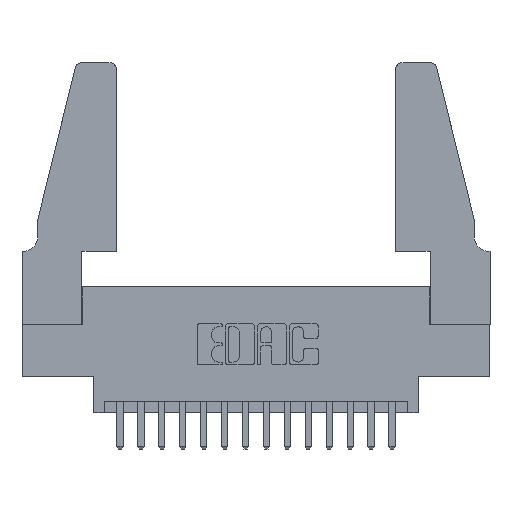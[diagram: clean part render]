
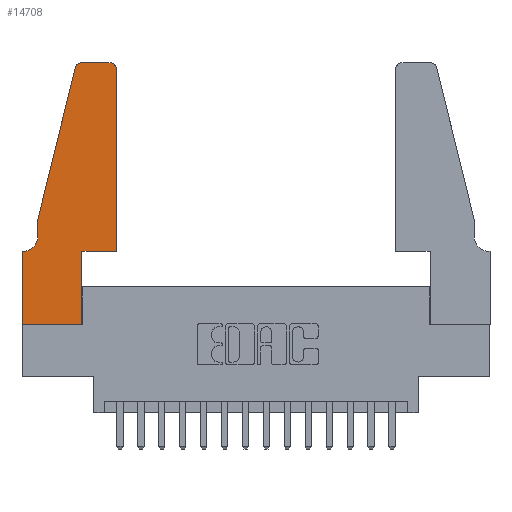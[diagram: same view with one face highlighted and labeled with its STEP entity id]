
A CAD part, top view. The second image highlights one B-rep face of the part: STEP entity #14708.
In plain terms, the highlighted planar face has unit normal (0, 0, 1).
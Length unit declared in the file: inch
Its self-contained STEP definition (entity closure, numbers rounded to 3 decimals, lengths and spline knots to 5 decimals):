
#23 = CARTESIAN_POINT ( 'NONE',  ( 0., 0., 0.37 ) ) ;
#335 = DIRECTION ( 'NONE',  ( 0., -1., 0. ) ) ;
#451 = DIRECTION ( 'NONE',  ( 0., 0., 1. ) ) ;
#635 = DIRECTION ( 'NONE',  ( 1., 0., 0. ) ) ;
#839 = VECTOR ( 'NONE', #14097, 39.37008 ) ;
#884 = EDGE_CURVE ( 'NONE', #7065, #16077, #8301, .T. ) ;
#1606 = EDGE_CURVE ( 'NONE', #11437, #7065, #13907, .T. ) ;
#1906 = LINE ( 'NONE', #2422, #11010 ) ;
#1949 = VERTEX_POINT ( 'NONE', #14188 ) ;
#2036 = VECTOR ( 'NONE', #12861, 39.37008 ) ;
#2192 = VERTEX_POINT ( 'NONE', #7810 ) ;
#2422 = CARTESIAN_POINT ( 'NONE',  ( 0.4505, 0.35, 0.37 ) ) ;
#2704 = ORIENTED_EDGE ( 'NONE', *, *, #884, .T. ) ;
#2797 = VECTOR ( 'NONE', #335, 39.37008 ) ;
#2861 = EDGE_CURVE ( 'NONE', #9238, #14686, #3278, .T. ) ;
#2967 = DIRECTION ( 'NONE',  ( -1., 0., 0. ) ) ;
#3145 = ORIENTED_EDGE ( 'NONE', *, *, #15824, .T. ) ;
#3198 = ORIENTED_EDGE ( 'NONE', *, *, #16057, .T. ) ;
#3278 = LINE ( 'NONE', #23, #9080 ) ;
#3473 = FACE_OUTER_BOUND ( 'NONE', #16788, .T. ) ;
#3894 = AXIS2_PLACEMENT_3D ( 'NONE', #6261, #12742, #635 ) ;
#3947 = DIRECTION ( 'NONE',  ( 1., 0., 0. ) ) ;
#4246 = ORIENTED_EDGE ( 'NONE', *, *, #7067, .T. ) ;
#4311 = LINE ( 'NONE', #10123, #839 ) ;
#4368 = EDGE_CURVE ( 'NONE', #16077, #9803, #7746, .T. ) ;
#4452 = ORIENTED_EDGE ( 'NONE', *, *, #8597, .T. ) ;
#4486 = LINE ( 'NONE', #6154, #2036 ) ;
#4610 = CARTESIAN_POINT ( 'NONE',  ( 0.0755, 0.42, 0.37 ) ) ;
#4617 = ORIENTED_EDGE ( 'NONE', *, *, #12117, .T. ) ;
#4648 = LINE ( 'NONE', #7163, #2797 ) ;
#4966 = CARTESIAN_POINT ( 'NONE',  ( 0.4205, 1.22, 0.37 ) ) ;
#5125 = CARTESIAN_POINT ( 'NONE',  ( 0.0755, 0.5, 0.37 ) ) ;
#5257 = DIRECTION ( 'NONE',  ( -1., 0., 0. ) ) ;
#5378 = EDGE_CURVE ( 'NONE', #6603, #6320, #1906, .T. ) ;
#5392 = VECTOR ( 'NONE', #6879, 39.37008 ) ;
#5452 = CARTESIAN_POINT ( 'NONE',  ( 0., 0.35, 0.37 ) ) ;
#5822 = DIRECTION ( 'NONE',  ( 0., 0., -1. ) ) ;
#5879 = CIRCLE ( 'NONE', #15345, 0.03 ) ;
#6154 = CARTESIAN_POINT ( 'NONE',  ( 0.0755, 0.5, 0.37 ) ) ;
#6238 = CARTESIAN_POINT ( 'NONE',  ( 0., 0., 0.37 ) ) ;
#6261 = CARTESIAN_POINT ( 'NONE',  ( 0., 0.35, 0.37 ) ) ;
#6320 = VERTEX_POINT ( 'NONE', #14788 ) ;
#6603 = VERTEX_POINT ( 'NONE', #6915 ) ;
#6679 = VECTOR ( 'NONE', #11986, 39.37008 ) ;
#6726 = VECTOR ( 'NONE', #13954, 39.37008 ) ;
#6879 = DIRECTION ( 'NONE',  ( 0., -1., 0. ) ) ;
#6915 = CARTESIAN_POINT ( 'NONE',  ( 0.4505, 0.35, 0.37 ) ) ;
#7061 = CARTESIAN_POINT ( 'NONE',  ( 0.25487, 1.22718, 0.37 ) ) ;
#7065 = VERTEX_POINT ( 'NONE', #4610 ) ;
#7067 = EDGE_CURVE ( 'NONE', #10405, #6603, #4311, .T. ) ;
#7163 = CARTESIAN_POINT ( 'NONE',  ( 0., 0., 0.37 ) ) ;
#7501 = CARTESIAN_POINT ( 'NONE',  ( 0.0055, 0.35, 0.37 ) ) ;
#7685 = PLANE ( 'NONE',  #3894 ) ;
#7728 = CIRCLE ( 'NONE', #14679, 0.03 ) ;
#7746 = LINE ( 'NONE', #10469, #10426 ) ;
#7810 = CARTESIAN_POINT ( 'NONE',  ( 0.4205, 1.25, 0.37 ) ) ;
#8301 = CIRCLE ( 'NONE', #9513, 0.07 ) ;
#8532 = ORIENTED_EDGE ( 'NONE', *, *, #1606, .T. ) ;
#8552 = CARTESIAN_POINT ( 'NONE',  ( 0.0755, 0.5, 0.37 ) ) ;
#8597 = EDGE_CURVE ( 'NONE', #11282, #11437, #4486, .T. ) ;
#9028 = DIRECTION ( 'NONE',  ( 0., 1., 0. ) ) ;
#9080 = VECTOR ( 'NONE', #3947, 39.37008 ) ;
#9238 = VERTEX_POINT ( 'NONE', #6238 ) ;
#9502 = ORIENTED_EDGE ( 'NONE', *, *, #10986, .T. ) ;
#9513 = AXIS2_PLACEMENT_3D ( 'NONE', #11075, #5822, #2967 ) ;
#9782 = CARTESIAN_POINT ( 'NONE',  ( 0.284, 1.22, 0.37 ) ) ;
#9803 = VERTEX_POINT ( 'NONE', #5452 ) ;
#10123 = CARTESIAN_POINT ( 'NONE',  ( 0.4505, 0.35, 0.37 ) ) ;
#10187 = LINE ( 'NONE', #10532, #6679 ) ;
#10405 = VERTEX_POINT ( 'NONE', #11746 ) ;
#10426 = VECTOR ( 'NONE', #5257, 39.37008 ) ;
#10469 = CARTESIAN_POINT ( 'NONE',  ( 0.0755, 0.35, 0.37 ) ) ;
#10532 = CARTESIAN_POINT ( 'NONE',  ( 0.2865, 0.35, 0.37 ) ) ;
#10986 = EDGE_CURVE ( 'NONE', #6320, #2192, #5879, .T. ) ;
#11010 = VECTOR ( 'NONE', #9028, 39.37008 ) ;
#11075 = CARTESIAN_POINT ( 'NONE',  ( 0.0055, 0.42, 0.37 ) ) ;
#11248 = EDGE_CURVE ( 'NONE', #1949, #11282, #7728, .T. ) ;
#11282 = VERTEX_POINT ( 'NONE', #7061 ) ;
#11437 = VERTEX_POINT ( 'NONE', #8552 ) ;
#11542 = CARTESIAN_POINT ( 'NONE',  ( 0.2865, 0., 0.37 ) ) ;
#11746 = CARTESIAN_POINT ( 'NONE',  ( 0.2865, 0.35, 0.37 ) ) ;
#11986 = DIRECTION ( 'NONE',  ( 0., 1., 0. ) ) ;
#12081 = ORIENTED_EDGE ( 'NONE', *, *, #11248, .T. ) ;
#12117 = EDGE_CURVE ( 'NONE', #14686, #10405, #10187, .T. ) ;
#12661 = CARTESIAN_POINT ( 'NONE',  ( 0.2605, 1.25, 0.37 ) ) ;
#12742 = DIRECTION ( 'NONE',  ( 0., 0., 1. ) ) ;
#12861 = DIRECTION ( 'NONE',  ( -0.239, -0.971, 0. ) ) ;
#13899 = ORIENTED_EDGE ( 'NONE', *, *, #5378, .T. ) ;
#13907 = LINE ( 'NONE', #5125, #5392 ) ;
#13954 = DIRECTION ( 'NONE',  ( -1., 0., 0. ) ) ;
#14097 = DIRECTION ( 'NONE',  ( 1., 0., 0. ) ) ;
#14188 = CARTESIAN_POINT ( 'NONE',  ( 0.284, 1.25, 0.37 ) ) ;
#14205 = LINE ( 'NONE', #12661, #6726 ) ;
#14273 = DIRECTION ( 'NONE',  ( 0., 0., 1. ) ) ;
#14328 = DIRECTION ( 'NONE',  ( 1., 0., 0. ) ) ;
#14670 = ORIENTED_EDGE ( 'NONE', *, *, #2861, .T. ) ;
#14679 = AXIS2_PLACEMENT_3D ( 'NONE', #9782, #451, #16244 ) ;
#14686 = VERTEX_POINT ( 'NONE', #11542 ) ;
#14708 = ADVANCED_FACE ( 'NONE', ( #3473 ), #7685, .T. ) ;
#14788 = CARTESIAN_POINT ( 'NONE',  ( 0.4505, 1.22, 0.37 ) ) ;
#15345 = AXIS2_PLACEMENT_3D ( 'NONE', #4966, #14273, #14328 ) ;
#15824 = EDGE_CURVE ( 'NONE', #9803, #9238, #4648, .T. ) ;
#16057 = EDGE_CURVE ( 'NONE', #2192, #1949, #14205, .T. ) ;
#16077 = VERTEX_POINT ( 'NONE', #7501 ) ;
#16244 = DIRECTION ( 'NONE',  ( 1., 0., 0. ) ) ;
#16513 = ORIENTED_EDGE ( 'NONE', *, *, #4368, .T. ) ;
#16788 = EDGE_LOOP ( 'NONE', ( #3198, #12081, #4452, #8532, #2704, #16513, #3145, #14670, #4617, #4246, #13899, #9502 ) ) ;
